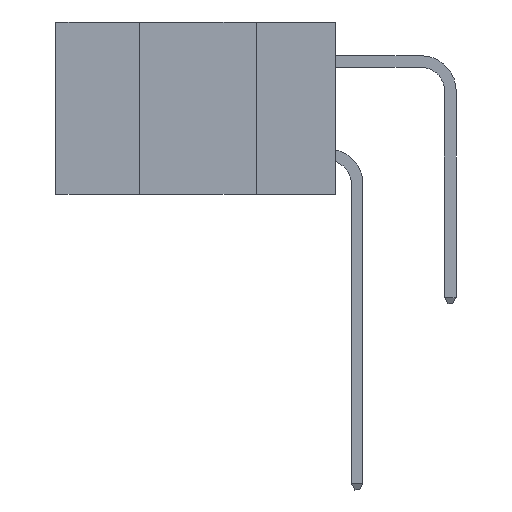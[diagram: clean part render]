
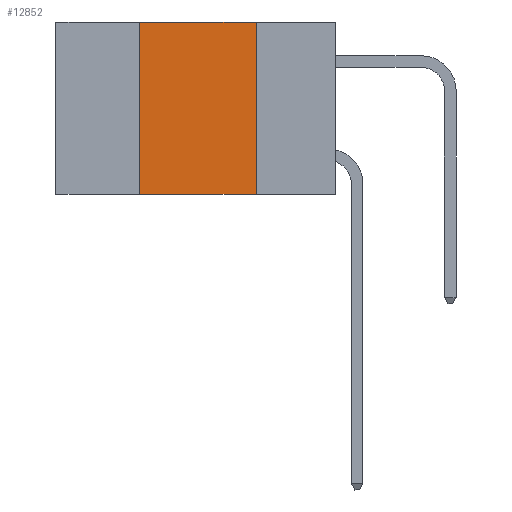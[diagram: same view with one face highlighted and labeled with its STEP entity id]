
A CAD part, left-side view. The second image highlights one B-rep face of the part: STEP entity #12852.
In plain terms, the highlighted planar face has unit normal (-1, 0, 0).
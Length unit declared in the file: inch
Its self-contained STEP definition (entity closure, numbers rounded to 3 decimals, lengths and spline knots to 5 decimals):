
#279 = DIRECTION ( 'NONE',  ( 0., -1., 0. ) ) ;
#435 = VECTOR ( 'NONE', #2066, 39.37008 ) ;
#737 = CARTESIAN_POINT ( 'NONE',  ( 0., 0.6, 0. ) ) ;
#1822 = VERTEX_POINT ( 'NONE', #13721 ) ;
#1836 = FACE_OUTER_BOUND ( 'NONE', #7286, .T. ) ;
#1878 = DIRECTION ( 'NONE',  ( 0., 0., -1. ) ) ;
#2066 = DIRECTION ( 'NONE',  ( 0., -1., 0. ) ) ;
#2550 = VECTOR ( 'NONE', #9331, 39.37008 ) ;
#2739 = CARTESIAN_POINT ( 'NONE',  ( 0., 0.42, -0.37 ) ) ;
#2873 = CARTESIAN_POINT ( 'NONE',  ( 0., 0.17, 0. ) ) ;
#3699 = CARTESIAN_POINT ( 'NONE',  ( 0., 0.42, 0. ) ) ;
#3728 = VECTOR ( 'NONE', #4823, 39.37008 ) ;
#4097 = ORIENTED_EDGE ( 'NONE', *, *, #8031, .F. ) ;
#4589 = ORIENTED_EDGE ( 'NONE', *, *, #11897, .F. ) ;
#4595 = VECTOR ( 'NONE', #279, 39.37008 ) ;
#4823 = DIRECTION ( 'NONE',  ( 0., 0., 1. ) ) ;
#5267 = VERTEX_POINT ( 'NONE', #2739 ) ;
#5565 = LINE ( 'NONE', #11518, #2550 ) ;
#5942 = CARTESIAN_POINT ( 'NONE',  ( 0., 0.6, -0.37 ) ) ;
#5998 = VERTEX_POINT ( 'NONE', #2873 ) ;
#6135 = ORIENTED_EDGE ( 'NONE', *, *, #11635, .F. ) ;
#6753 = AXIS2_PLACEMENT_3D ( 'NONE', #737, #8652, #1878 ) ;
#7017 = CARTESIAN_POINT ( 'NONE',  ( 0., 0.42, 0. ) ) ;
#7286 = EDGE_LOOP ( 'NONE', ( #4589, #6135, #4097, #12149 ) ) ;
#7501 = PLANE ( 'NONE',  #6753 ) ;
#7619 = LINE ( 'NONE', #5942, #4595 ) ;
#8019 = EDGE_CURVE ( 'NONE', #5267, #1822, #7619, .T. ) ;
#8031 = EDGE_CURVE ( 'NONE', #5267, #12563, #13491, .T. ) ;
#8652 = DIRECTION ( 'NONE',  ( 1., 0., 0. ) ) ;
#8841 = CARTESIAN_POINT ( 'NONE',  ( 0., 0.6, 0. ) ) ;
#9331 = DIRECTION ( 'NONE',  ( 0., 0., -1. ) ) ;
#9440 = LINE ( 'NONE', #8841, #435 ) ;
#11518 = CARTESIAN_POINT ( 'NONE',  ( 0., 0.17, 0. ) ) ;
#11635 = EDGE_CURVE ( 'NONE', #12563, #5998, #9440, .T. ) ;
#11897 = EDGE_CURVE ( 'NONE', #5998, #1822, #5565, .T. ) ;
#12149 = ORIENTED_EDGE ( 'NONE', *, *, #8019, .T. ) ;
#12563 = VERTEX_POINT ( 'NONE', #7017 ) ;
#12852 = ADVANCED_FACE ( 'NONE', ( #1836 ), #7501, .F. ) ;
#13491 = LINE ( 'NONE', #3699, #3728 ) ;
#13721 = CARTESIAN_POINT ( 'NONE',  ( 0., 0.17, -0.37 ) ) ;
